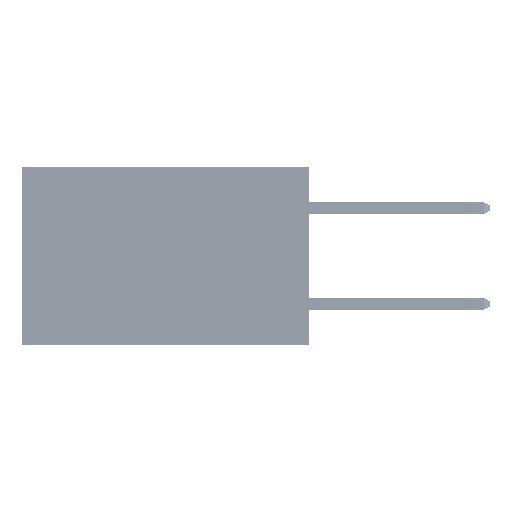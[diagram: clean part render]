
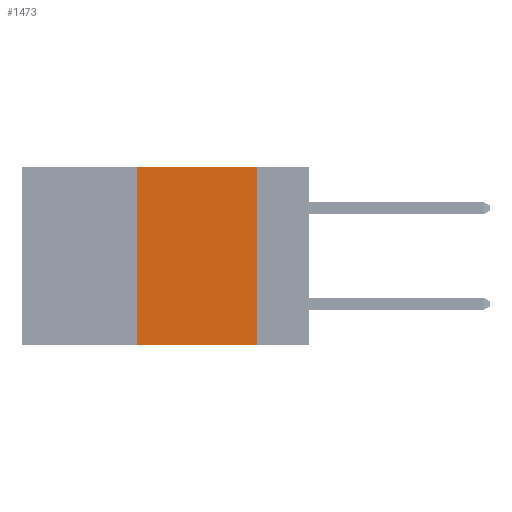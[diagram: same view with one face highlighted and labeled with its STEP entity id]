
A CAD part, left-side view. The second image highlights one B-rep face of the part: STEP entity #1473.
In plain terms, the highlighted planar face has unit normal (-1, 0, 0).
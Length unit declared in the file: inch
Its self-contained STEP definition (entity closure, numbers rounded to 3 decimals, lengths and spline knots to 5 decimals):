
#67 = VERTEX_POINT ( 'NONE', #3439 ) ;
#198 = DIRECTION ( 'NONE',  ( 1., 0., 0. ) ) ;
#254 = ORIENTED_EDGE ( 'NONE', *, *, #39902, .T. ) ;
#534 = DIRECTION ( 'NONE',  ( 0., 0., 1. ) ) ;
#1151 = ORIENTED_EDGE ( 'NONE', *, *, #19938, .F. ) ;
#1473 = ADVANCED_FACE ( 'NONE', ( #45013 ), #30296, .F. ) ;
#1708 = VERTEX_POINT ( 'NONE', #32021 ) ;
#3439 = CARTESIAN_POINT ( 'NONE',  ( 0., 0.36, -0.37 ) ) ;
#4276 = CARTESIAN_POINT ( 'NONE',  ( 0., 0.36, 0. ) ) ;
#4631 = LINE ( 'NONE', #31247, #47674 ) ;
#5360 = DIRECTION ( 'NONE',  ( 0., -1., 0. ) ) ;
#8468 = VERTEX_POINT ( 'NONE', #17767 ) ;
#9224 = EDGE_CURVE ( 'NONE', #67, #8468, #23148, .T. ) ;
#10091 = VECTOR ( 'NONE', #43087, 39.37008 ) ;
#10915 = CARTESIAN_POINT ( 'NONE',  ( 0., 0.6, 0. ) ) ;
#12698 = DIRECTION ( 'NONE',  ( 0., -1., 0. ) ) ;
#12725 = LINE ( 'NONE', #27889, #10091 ) ;
#15375 = DIRECTION ( 'NONE',  ( 0., 0., -1. ) ) ;
#16060 = VECTOR ( 'NONE', #12698, 39.37008 ) ;
#17767 = CARTESIAN_POINT ( 'NONE',  ( 0., 0.36, 0. ) ) ;
#19938 = EDGE_CURVE ( 'NONE', #24505, #1708, #12725, .T. ) ;
#23148 = LINE ( 'NONE', #4276, #32374 ) ;
#23626 = CARTESIAN_POINT ( 'NONE',  ( 0., 0.6, 0. ) ) ;
#23865 = LINE ( 'NONE', #23626, #16060 ) ;
#24505 = VERTEX_POINT ( 'NONE', #46904 ) ;
#26603 = EDGE_CURVE ( 'NONE', #8468, #24505, #23865, .T. ) ;
#27889 = CARTESIAN_POINT ( 'NONE',  ( 0., 0.11, 0. ) ) ;
#30296 = PLANE ( 'NONE',  #48303 ) ;
#31247 = CARTESIAN_POINT ( 'NONE',  ( 0., 0.6, -0.37 ) ) ;
#32021 = CARTESIAN_POINT ( 'NONE',  ( 0., 0.11, -0.37 ) ) ;
#32374 = VECTOR ( 'NONE', #534, 39.37008 ) ;
#38548 = ORIENTED_EDGE ( 'NONE', *, *, #26603, .F. ) ;
#39902 = EDGE_CURVE ( 'NONE', #67, #1708, #4631, .T. ) ;
#41922 = EDGE_LOOP ( 'NONE', ( #1151, #38548, #44103, #254 ) ) ;
#43087 = DIRECTION ( 'NONE',  ( 0., 0., -1. ) ) ;
#44103 = ORIENTED_EDGE ( 'NONE', *, *, #9224, .F. ) ;
#45013 = FACE_OUTER_BOUND ( 'NONE', #41922, .T. ) ;
#46904 = CARTESIAN_POINT ( 'NONE',  ( 0., 0.11, 0. ) ) ;
#47674 = VECTOR ( 'NONE', #5360, 39.37008 ) ;
#48303 = AXIS2_PLACEMENT_3D ( 'NONE', #10915, #198, #15375 ) ;
